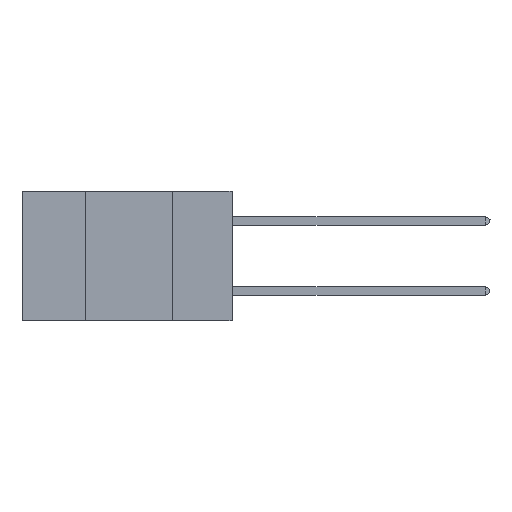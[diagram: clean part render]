
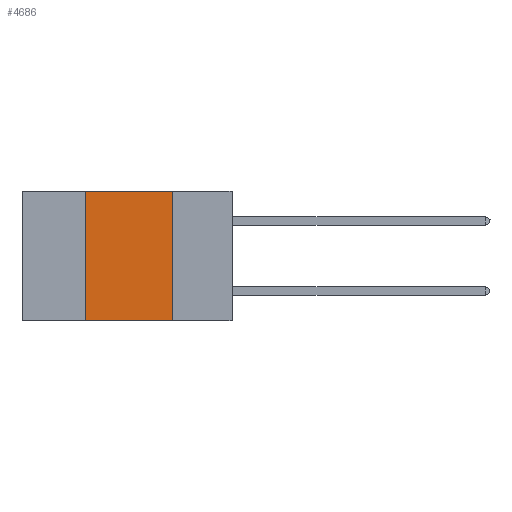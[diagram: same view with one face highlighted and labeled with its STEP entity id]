
A CAD part, left-side view. The second image highlights one B-rep face of the part: STEP entity #4686.
In plain terms, the highlighted planar face has unit normal (-1, 0, 0).
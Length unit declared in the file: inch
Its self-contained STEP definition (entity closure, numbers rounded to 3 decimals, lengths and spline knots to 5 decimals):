
#295 = VERTEX_POINT ( 'NONE', #1724 ) ;
#453 = VERTEX_POINT ( 'NONE', #13099 ) ;
#591 = LINE ( 'NONE', #16446, #13386 ) ;
#650 = VERTEX_POINT ( 'NONE', #12501 ) ;
#929 = DIRECTION ( 'NONE',  ( 0., 0., 1. ) ) ;
#1103 = DIRECTION ( 'NONE',  ( 1., 0., 0. ) ) ;
#1193 = LINE ( 'NONE', #17214, #7375 ) ;
#1724 = CARTESIAN_POINT ( 'NONE',  ( 0., 0.42, 0. ) ) ;
#2260 = LINE ( 'NONE', #7614, #11100 ) ;
#3186 = ORIENTED_EDGE ( 'NONE', *, *, #13844, .F. ) ;
#4003 = CARTESIAN_POINT ( 'NONE',  ( 0., 0.6, 0. ) ) ;
#4264 = EDGE_LOOP ( 'NONE', ( #16522, #3186, #8938, #5544 ) ) ;
#4475 = EDGE_CURVE ( 'NONE', #650, #453, #591, .T. ) ;
#4686 = ADVANCED_FACE ( 'NONE', ( #14574 ), #10413, .F. ) ;
#4750 = EDGE_CURVE ( 'NONE', #12329, #453, #1193, .T. ) ;
#5544 = ORIENTED_EDGE ( 'NONE', *, *, #4750, .T. ) ;
#6300 = CARTESIAN_POINT ( 'NONE',  ( 0., 0.6, 0. ) ) ;
#7375 = VECTOR ( 'NONE', #14319, 39.37008 ) ;
#7614 = CARTESIAN_POINT ( 'NONE',  ( 0., 0.42, 0. ) ) ;
#8325 = DIRECTION ( 'NONE',  ( 0., -1., 0. ) ) ;
#8938 = ORIENTED_EDGE ( 'NONE', *, *, #17119, .F. ) ;
#9944 = AXIS2_PLACEMENT_3D ( 'NONE', #6300, #1103, #15710 ) ;
#10413 = PLANE ( 'NONE',  #9944 ) ;
#10761 = LINE ( 'NONE', #4003, #14393 ) ;
#11100 = VECTOR ( 'NONE', #929, 39.37008 ) ;
#11479 = DIRECTION ( 'NONE',  ( 0., 0., -1. ) ) ;
#11486 = CARTESIAN_POINT ( 'NONE',  ( 0., 0.42, -0.37 ) ) ;
#12329 = VERTEX_POINT ( 'NONE', #11486 ) ;
#12501 = CARTESIAN_POINT ( 'NONE',  ( 0., 0.17, 0. ) ) ;
#13099 = CARTESIAN_POINT ( 'NONE',  ( 0., 0.17, -0.37 ) ) ;
#13386 = VECTOR ( 'NONE', #11479, 39.37008 ) ;
#13844 = EDGE_CURVE ( 'NONE', #295, #650, #10761, .T. ) ;
#14319 = DIRECTION ( 'NONE',  ( 0., -1., 0. ) ) ;
#14393 = VECTOR ( 'NONE', #8325, 39.37008 ) ;
#14574 = FACE_OUTER_BOUND ( 'NONE', #4264, .T. ) ;
#15710 = DIRECTION ( 'NONE',  ( 0., 0., -1. ) ) ;
#16446 = CARTESIAN_POINT ( 'NONE',  ( 0., 0.17, 0. ) ) ;
#16522 = ORIENTED_EDGE ( 'NONE', *, *, #4475, .F. ) ;
#17119 = EDGE_CURVE ( 'NONE', #12329, #295, #2260, .T. ) ;
#17214 = CARTESIAN_POINT ( 'NONE',  ( 0., 0.6, -0.37 ) ) ;
